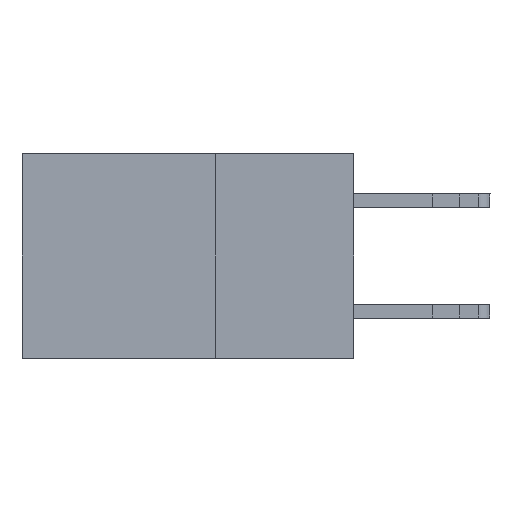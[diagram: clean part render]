
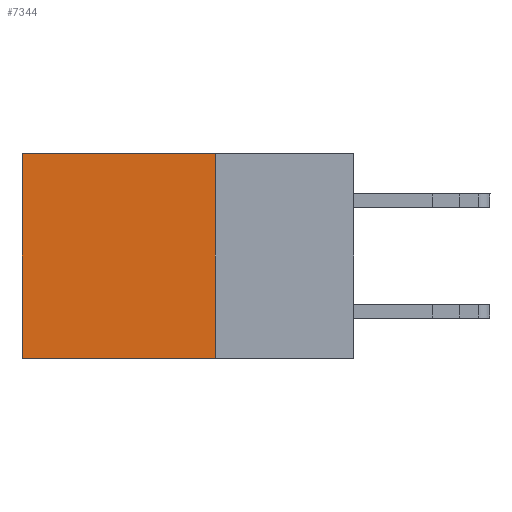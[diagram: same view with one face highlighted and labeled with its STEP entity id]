
A CAD part, left-side view. The second image highlights one B-rep face of the part: STEP entity #7344.
In plain terms, the highlighted planar face has unit normal (-1, 0, 0).
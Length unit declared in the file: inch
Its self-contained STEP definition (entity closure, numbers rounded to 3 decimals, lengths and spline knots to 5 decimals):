
#3743 = DIRECTION ( 'NONE',  ( 0., 1., 0. ) ) ;
#4420 = VERTEX_POINT ( 'NONE', #20380 ) ;
#4908 = FACE_OUTER_BOUND ( 'NONE', #23732, .T. ) ;
#6899 = CARTESIAN_POINT ( 'NONE',  ( 0.2875, 0.25, 0. ) ) ;
#7246 = VERTEX_POINT ( 'NONE', #26996 ) ;
#7344 = ADVANCED_FACE ( 'NONE', ( #4908 ), #29491, .F. ) ;
#9291 = CARTESIAN_POINT ( 'NONE',  ( 0.2875, 0.25, 0. ) ) ;
#9999 = VECTOR ( 'NONE', #21775, 39.37008 ) ;
#13977 = CARTESIAN_POINT ( 'NONE',  ( 0.2875, 0.6, 0. ) ) ;
#15224 = VECTOR ( 'NONE', #3743, 39.37008 ) ;
#15802 = EDGE_CURVE ( 'NONE', #17012, #18972, #25318, .T. ) ;
#16135 = CARTESIAN_POINT ( 'NONE',  ( 0.2875, 0.25, 0. ) ) ;
#16787 = EDGE_CURVE ( 'NONE', #7246, #4420, #18666, .T. ) ;
#16898 = ORIENTED_EDGE ( 'NONE', *, *, #17704, .F. ) ;
#16929 = DIRECTION ( 'NONE',  ( 0., 0., -1. ) ) ;
#16948 = LINE ( 'NONE', #31324, #29336 ) ;
#17012 = VERTEX_POINT ( 'NONE', #17756 ) ;
#17704 = EDGE_CURVE ( 'NONE', #17012, #7246, #29495, .T. ) ;
#17756 = CARTESIAN_POINT ( 'NONE',  ( 0.2875, 0.25, 0. ) ) ;
#18666 = LINE ( 'NONE', #20683, #15224 ) ;
#18724 = VECTOR ( 'NONE', #31179, 39.37008 ) ;
#18903 = ORIENTED_EDGE ( 'NONE', *, *, #22562, .T. ) ;
#18972 = VERTEX_POINT ( 'NONE', #13977 ) ;
#20380 = CARTESIAN_POINT ( 'NONE',  ( 0.2875, 0.6, -0.37 ) ) ;
#20683 = CARTESIAN_POINT ( 'NONE',  ( 0.2875, 0.25, -0.37 ) ) ;
#21775 = DIRECTION ( 'NONE',  ( 0., 0., -1. ) ) ;
#22562 = EDGE_CURVE ( 'NONE', #18972, #4420, #16948, .T. ) ;
#23732 = EDGE_LOOP ( 'NONE', ( #18903, #32222, #16898, #29855 ) ) ;
#24539 = DIRECTION ( 'NONE',  ( 1., 0., 0. ) ) ;
#25048 = AXIS2_PLACEMENT_3D ( 'NONE', #6899, #24539, #16929 ) ;
#25318 = LINE ( 'NONE', #16135, #18724 ) ;
#26996 = CARTESIAN_POINT ( 'NONE',  ( 0.2875, 0.25, -0.37 ) ) ;
#29336 = VECTOR ( 'NONE', #29945, 39.37008 ) ;
#29491 = PLANE ( 'NONE',  #25048 ) ;
#29495 = LINE ( 'NONE', #9291, #9999 ) ;
#29855 = ORIENTED_EDGE ( 'NONE', *, *, #15802, .T. ) ;
#29945 = DIRECTION ( 'NONE',  ( 0., 0., -1. ) ) ;
#31179 = DIRECTION ( 'NONE',  ( 0., 1., 0. ) ) ;
#31324 = CARTESIAN_POINT ( 'NONE',  ( 0.2875, 0.6, 0. ) ) ;
#32222 = ORIENTED_EDGE ( 'NONE', *, *, #16787, .F. ) ;
